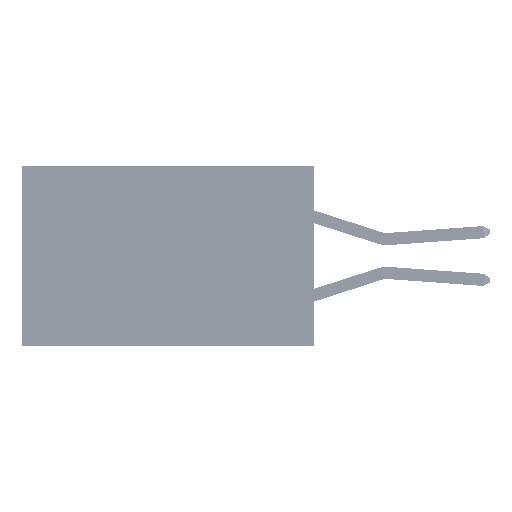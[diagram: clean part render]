
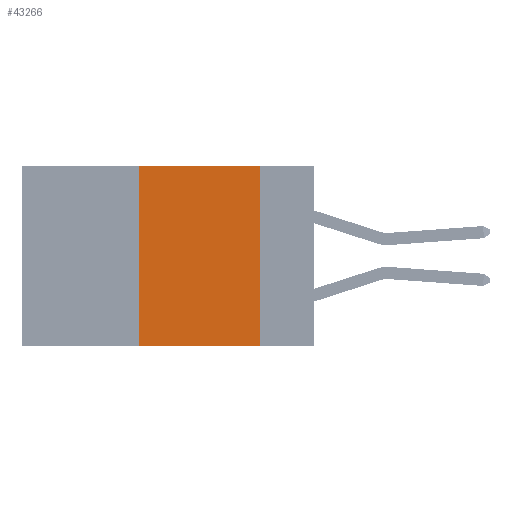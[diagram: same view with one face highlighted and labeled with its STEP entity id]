
A CAD part, left-side view. The second image highlights one B-rep face of the part: STEP entity #43266.
In plain terms, the highlighted planar face has unit normal (-1, 0, 0).
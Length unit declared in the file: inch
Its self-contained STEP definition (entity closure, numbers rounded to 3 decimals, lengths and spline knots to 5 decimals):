
#925 = ORIENTED_EDGE ( 'NONE', *, *, #3466, .F. ) ;
#3466 = EDGE_CURVE ( 'NONE', #38987, #24697, #22770, .T. ) ;
#4657 = CARTESIAN_POINT ( 'NONE',  ( 0., 0.36, -0.37 ) ) ;
#4756 = FACE_OUTER_BOUND ( 'NONE', #40204, .T. ) ;
#6981 = CARTESIAN_POINT ( 'NONE',  ( 0., 0.11, 0. ) ) ;
#7983 = ORIENTED_EDGE ( 'NONE', *, *, #44712, .F. ) ;
#8194 = VECTOR ( 'NONE', #46305, 39.37008 ) ;
#8941 = DIRECTION ( 'NONE',  ( 0., 0., -1. ) ) ;
#9252 = DIRECTION ( 'NONE',  ( 1., 0., 0. ) ) ;
#10284 = LINE ( 'NONE', #14644, #22922 ) ;
#11860 = ORIENTED_EDGE ( 'NONE', *, *, #18812, .F. ) ;
#14177 = EDGE_CURVE ( 'NONE', #20031, #24697, #26335, .T. ) ;
#14644 = CARTESIAN_POINT ( 'NONE',  ( 0., 0.36, 0. ) ) ;
#15368 = CARTESIAN_POINT ( 'NONE',  ( 0., 0.11, -0.37 ) ) ;
#18812 = EDGE_CURVE ( 'NONE', #41604, #38987, #35075, .T. ) ;
#20031 = VERTEX_POINT ( 'NONE', #4657 ) ;
#20733 = CARTESIAN_POINT ( 'NONE',  ( 0., 0.6, 0. ) ) ;
#21006 = ORIENTED_EDGE ( 'NONE', *, *, #14177, .T. ) ;
#22770 = LINE ( 'NONE', #6981, #25047 ) ;
#22922 = VECTOR ( 'NONE', #33219, 39.37008 ) ;
#24697 = VERTEX_POINT ( 'NONE', #15368 ) ;
#25047 = VECTOR ( 'NONE', #25685, 39.37008 ) ;
#25685 = DIRECTION ( 'NONE',  ( 0., 0., -1. ) ) ;
#26335 = LINE ( 'NONE', #39433, #36101 ) ;
#27483 = CARTESIAN_POINT ( 'NONE',  ( 0., 0.6, 0. ) ) ;
#32177 = CARTESIAN_POINT ( 'NONE',  ( 0., 0.36, 0. ) ) ;
#33219 = DIRECTION ( 'NONE',  ( 0., 0., 1. ) ) ;
#35075 = LINE ( 'NONE', #20733, #8194 ) ;
#36101 = VECTOR ( 'NONE', #36891, 39.37008 ) ;
#36891 = DIRECTION ( 'NONE',  ( 0., -1., 0. ) ) ;
#38392 = PLANE ( 'NONE',  #43892 ) ;
#38987 = VERTEX_POINT ( 'NONE', #44428 ) ;
#39433 = CARTESIAN_POINT ( 'NONE',  ( 0., 0.6, -0.37 ) ) ;
#40204 = EDGE_LOOP ( 'NONE', ( #925, #11860, #7983, #21006 ) ) ;
#41604 = VERTEX_POINT ( 'NONE', #32177 ) ;
#43266 = ADVANCED_FACE ( 'NONE', ( #4756 ), #38392, .F. ) ;
#43892 = AXIS2_PLACEMENT_3D ( 'NONE', #27483, #9252, #8941 ) ;
#44428 = CARTESIAN_POINT ( 'NONE',  ( 0., 0.11, 0. ) ) ;
#44712 = EDGE_CURVE ( 'NONE', #20031, #41604, #10284, .T. ) ;
#46305 = DIRECTION ( 'NONE',  ( 0., -1., 0. ) ) ;
